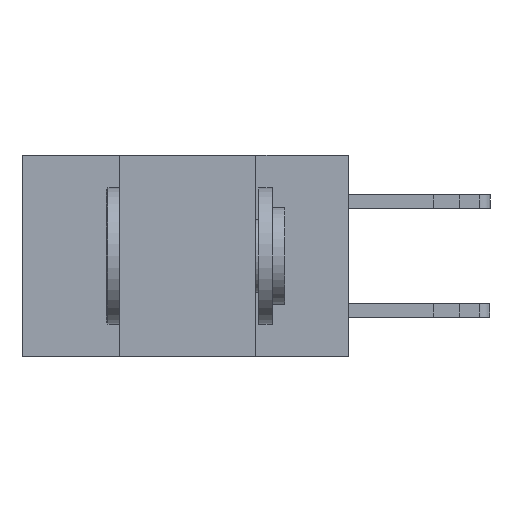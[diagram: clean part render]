
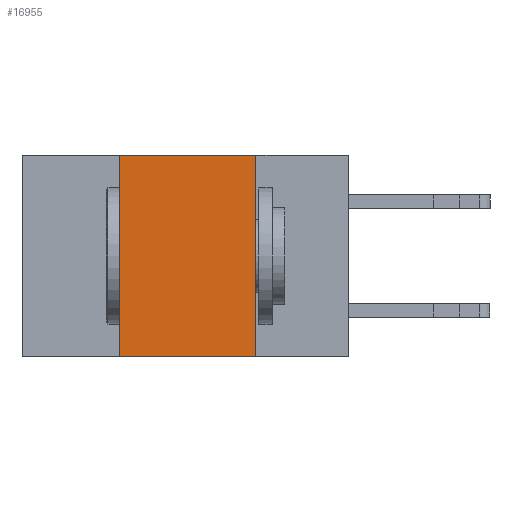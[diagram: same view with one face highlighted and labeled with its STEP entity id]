
A CAD part, left-side view. The second image highlights one B-rep face of the part: STEP entity #16955.
In plain terms, the highlighted planar face has unit normal (-1, 0, 0).
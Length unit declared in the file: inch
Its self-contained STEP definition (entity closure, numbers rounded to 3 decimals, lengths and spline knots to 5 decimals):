
#156 = VECTOR ( 'NONE', #4426, 39.37008 ) ;
#225 = CARTESIAN_POINT ( 'NONE',  ( 0., 0.6, 0. ) ) ;
#269 = CARTESIAN_POINT ( 'NONE',  ( 0., 0.6, 0. ) ) ;
#279 = LINE ( 'NONE', #6312, #13544 ) ;
#371 = EDGE_CURVE ( 'NONE', #3929, #18671, #12566, .T. ) ;
#473 = EDGE_LOOP ( 'NONE', ( #3770, #4876, #15713, #3509 ) ) ;
#2681 = CARTESIAN_POINT ( 'NONE',  ( 0., 0.17, 0. ) ) ;
#3337 = VERTEX_POINT ( 'NONE', #20003 ) ;
#3509 = ORIENTED_EDGE ( 'NONE', *, *, #11199, .T. ) ;
#3670 = DIRECTION ( 'NONE',  ( 0., -1., 0. ) ) ;
#3770 = ORIENTED_EDGE ( 'NONE', *, *, #17688, .F. ) ;
#3929 = VERTEX_POINT ( 'NONE', #16428 ) ;
#4426 = DIRECTION ( 'NONE',  ( 0., 0., -1. ) ) ;
#4876 = ORIENTED_EDGE ( 'NONE', *, *, #20565, .F. ) ;
#5674 = CARTESIAN_POINT ( 'NONE',  ( 0., 0.42, 0. ) ) ;
#6108 = DIRECTION ( 'NONE',  ( 0., 0., 1. ) ) ;
#6312 = CARTESIAN_POINT ( 'NONE',  ( 0., 0.6, -0.37 ) ) ;
#7192 = DIRECTION ( 'NONE',  ( 0., 0., -1. ) ) ;
#7817 = VECTOR ( 'NONE', #3670, 39.37008 ) ;
#8371 = LINE ( 'NONE', #225, #7817 ) ;
#9680 = CARTESIAN_POINT ( 'NONE',  ( 0., 0.17, -0.37 ) ) ;
#10821 = FACE_OUTER_BOUND ( 'NONE', #473, .T. ) ;
#11199 = EDGE_CURVE ( 'NONE', #3929, #17250, #279, .T. ) ;
#12315 = PLANE ( 'NONE',  #14195 ) ;
#12566 = LINE ( 'NONE', #16438, #16647 ) ;
#13422 = LINE ( 'NONE', #2681, #156 ) ;
#13544 = VECTOR ( 'NONE', #18714, 39.37008 ) ;
#14195 = AXIS2_PLACEMENT_3D ( 'NONE', #269, #17527, #7192 ) ;
#15713 = ORIENTED_EDGE ( 'NONE', *, *, #371, .F. ) ;
#16428 = CARTESIAN_POINT ( 'NONE',  ( 0., 0.42, -0.37 ) ) ;
#16438 = CARTESIAN_POINT ( 'NONE',  ( 0., 0.42, 0. ) ) ;
#16647 = VECTOR ( 'NONE', #6108, 39.37008 ) ;
#16955 = ADVANCED_FACE ( 'NONE', ( #10821 ), #12315, .F. ) ;
#17250 = VERTEX_POINT ( 'NONE', #9680 ) ;
#17527 = DIRECTION ( 'NONE',  ( 1., 0., 0. ) ) ;
#17688 = EDGE_CURVE ( 'NONE', #3337, #17250, #13422, .T. ) ;
#18671 = VERTEX_POINT ( 'NONE', #5674 ) ;
#18714 = DIRECTION ( 'NONE',  ( 0., -1., 0. ) ) ;
#20003 = CARTESIAN_POINT ( 'NONE',  ( 0., 0.17, 0. ) ) ;
#20565 = EDGE_CURVE ( 'NONE', #18671, #3337, #8371, .T. ) ;
